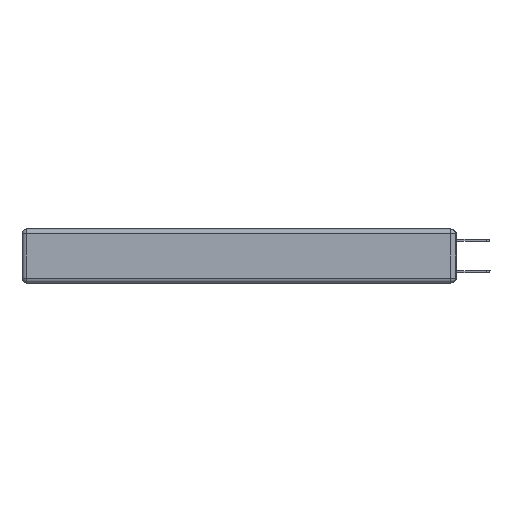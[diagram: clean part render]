
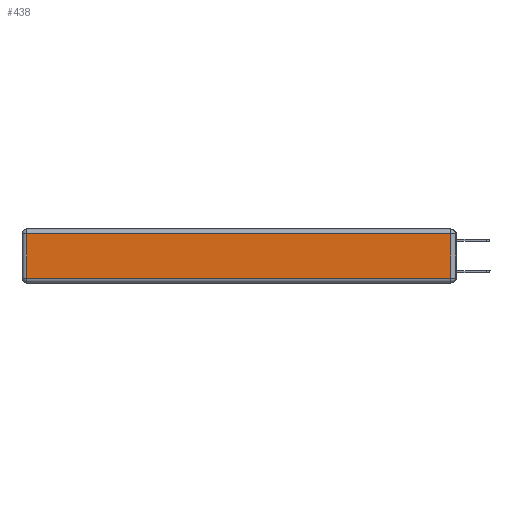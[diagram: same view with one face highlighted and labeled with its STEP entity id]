
A CAD part, left-side view. The second image highlights one B-rep face of the part: STEP entity #438.
In plain terms, the highlighted planar face has unit normal (-1, 0, 0).
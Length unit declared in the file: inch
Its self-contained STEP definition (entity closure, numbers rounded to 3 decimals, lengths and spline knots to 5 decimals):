
#438 = ADVANCED_FACE ( 'NONE', ( #17082 ), #3736, .T. ) ;
#1285 = EDGE_CURVE ( 'NONE', #4784, #6198, #19649, .T. ) ;
#1521 = VERTEX_POINT ( 'NONE', #21026 ) ;
#1630 = EDGE_CURVE ( 'NONE', #6198, #5979, #19912, .T. ) ;
#1849 = CARTESIAN_POINT ( 'NONE',  ( 0., 2.75, -0.03 ) ) ;
#2823 = LINE ( 'NONE', #1849, #13230 ) ;
#3439 = CARTESIAN_POINT ( 'NONE',  ( 0., 0.03, -0.313 ) ) ;
#3736 = PLANE ( 'NONE',  #21521 ) ;
#3983 = DIRECTION ( 'NONE',  ( -1., 0., 0. ) ) ;
#4561 = ORIENTED_EDGE ( 'NONE', *, *, #21574, .T. ) ;
#4784 = VERTEX_POINT ( 'NONE', #10967 ) ;
#4873 = DIRECTION ( 'NONE',  ( 0., -1., 0. ) ) ;
#5379 = EDGE_LOOP ( 'NONE', ( #22005, #15623, #4561, #6897 ) ) ;
#5979 = VERTEX_POINT ( 'NONE', #3439 ) ;
#6198 = VERTEX_POINT ( 'NONE', #10167 ) ;
#6897 = ORIENTED_EDGE ( 'NONE', *, *, #1285, .T. ) ;
#7764 = VECTOR ( 'NONE', #19271, 39.37008 ) ;
#10167 = CARTESIAN_POINT ( 'NONE',  ( 0., 2.72, -0.313 ) ) ;
#10967 = CARTESIAN_POINT ( 'NONE',  ( 0., 2.72, -0.03 ) ) ;
#11637 = DIRECTION ( 'NONE',  ( 0., 0., -1. ) ) ;
#13230 = VECTOR ( 'NONE', #20068, 39.37008 ) ;
#15453 = CARTESIAN_POINT ( 'NONE',  ( 0., 2.72, -0.343 ) ) ;
#15623 = ORIENTED_EDGE ( 'NONE', *, *, #21834, .T. ) ;
#17082 = FACE_OUTER_BOUND ( 'NONE', #5379, .T. ) ;
#18629 = CARTESIAN_POINT ( 'NONE',  ( 0., 0., -0.343 ) ) ;
#19271 = DIRECTION ( 'NONE',  ( 0., 0., 1. ) ) ;
#19649 = LINE ( 'NONE', #15453, #23123 ) ;
#19912 = LINE ( 'NONE', #21761, #21947 ) ;
#20068 = DIRECTION ( 'NONE',  ( 0., 1., 0. ) ) ;
#20184 = LINE ( 'NONE', #21021, #7764 ) ;
#20468 = DIRECTION ( 'NONE',  ( 0., 0., 1. ) ) ;
#21021 = CARTESIAN_POINT ( 'NONE',  ( 0., 0.03, -0.343 ) ) ;
#21026 = CARTESIAN_POINT ( 'NONE',  ( 0., 0.03, -0.03 ) ) ;
#21521 = AXIS2_PLACEMENT_3D ( 'NONE', #18629, #3983, #20468 ) ;
#21574 = EDGE_CURVE ( 'NONE', #1521, #4784, #2823, .T. ) ;
#21761 = CARTESIAN_POINT ( 'NONE',  ( 0., 0., -0.313 ) ) ;
#21834 = EDGE_CURVE ( 'NONE', #5979, #1521, #20184, .T. ) ;
#21947 = VECTOR ( 'NONE', #4873, 39.37008 ) ;
#22005 = ORIENTED_EDGE ( 'NONE', *, *, #1630, .T. ) ;
#23123 = VECTOR ( 'NONE', #11637, 39.37008 ) ;
